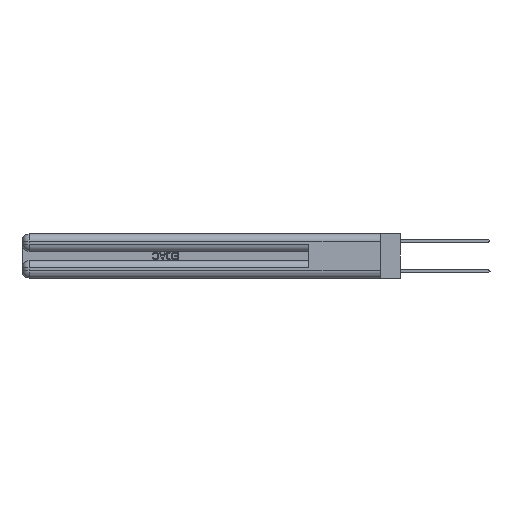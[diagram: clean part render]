
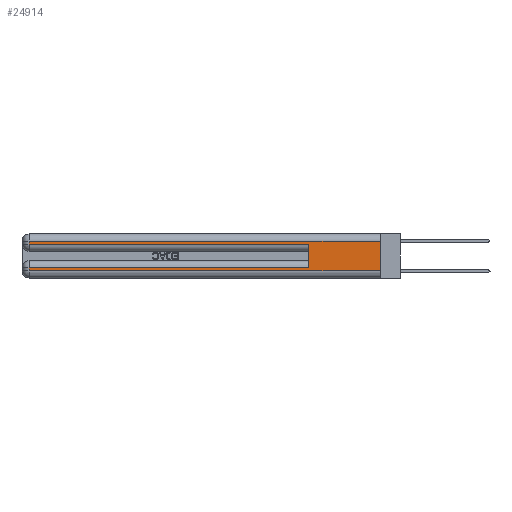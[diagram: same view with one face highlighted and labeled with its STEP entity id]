
A CAD part, left-side view. The second image highlights one B-rep face of the part: STEP entity #24914.
In plain terms, the highlighted planar face has unit normal (-1, 0, 0).
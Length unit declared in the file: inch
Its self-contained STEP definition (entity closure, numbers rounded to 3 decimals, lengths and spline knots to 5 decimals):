
#585 = EDGE_CURVE ( 'NONE', #25290, #20435, #10890, .T. ) ;
#589 = ORIENTED_EDGE ( 'NONE', *, *, #7369, .T. ) ;
#964 = CARTESIAN_POINT ( 'NONE',  ( 0., 0., 0.37 ) ) ;
#1175 = DIRECTION ( 'NONE',  ( 0., 0., -1. ) ) ;
#1409 = LINE ( 'NONE', #19033, #17238 ) ;
#1501 = LINE ( 'NONE', #21539, #28859 ) ;
#2198 = DIRECTION ( 'NONE',  ( 0., 1., 0. ) ) ;
#2528 = CARTESIAN_POINT ( 'NONE',  ( 0., 2.94, 0.06 ) ) ;
#3525 = ORIENTED_EDGE ( 'NONE', *, *, #28565, .T. ) ;
#4118 = CARTESIAN_POINT ( 'NONE',  ( 0., 2.94, 0.37 ) ) ;
#4398 = DIRECTION ( 'NONE',  ( 0., -1., 0. ) ) ;
#4461 = AXIS2_PLACEMENT_3D ( 'NONE', #27944, #15778, #1175 ) ;
#4670 = DIRECTION ( 'NONE',  ( 0., 0., 1. ) ) ;
#5052 = VERTEX_POINT ( 'NONE', #25708 ) ;
#5996 = FACE_OUTER_BOUND ( 'NONE', #27576, .T. ) ;
#6128 = LINE ( 'NONE', #26001, #10800 ) ;
#6422 = CARTESIAN_POINT ( 'NONE',  ( 0., 0., 0.31 ) ) ;
#6440 = DIRECTION ( 'NONE',  ( 0., 0., -1. ) ) ;
#7369 = EDGE_CURVE ( 'NONE', #26856, #5052, #14065, .T. ) ;
#7680 = VECTOR ( 'NONE', #4670, 39.37008 ) ;
#8380 = PLANE ( 'NONE',  #4461 ) ;
#8761 = CARTESIAN_POINT ( 'NONE',  ( 0., 0.6, 0.285 ) ) ;
#9055 = EDGE_CURVE ( 'NONE', #12530, #19710, #1501, .T. ) ;
#9085 = LINE ( 'NONE', #4118, #18811 ) ;
#9588 = EDGE_CURVE ( 'NONE', #26856, #19710, #29171, .T. ) ;
#9983 = EDGE_CURVE ( 'NONE', #5052, #23613, #9085, .T. ) ;
#10800 = VECTOR ( 'NONE', #6440, 39.37008 ) ;
#10890 = LINE ( 'NONE', #964, #15749 ) ;
#12530 = VERTEX_POINT ( 'NONE', #13041 ) ;
#13041 = CARTESIAN_POINT ( 'NONE',  ( 0., 2.94, 0.285 ) ) ;
#13114 = VECTOR ( 'NONE', #2198, 39.37008 ) ;
#13145 = CARTESIAN_POINT ( 'NONE',  ( 0., 0., 0.06 ) ) ;
#14011 = ORIENTED_EDGE ( 'NONE', *, *, #24035, .T. ) ;
#14065 = LINE ( 'NONE', #23860, #13114 ) ;
#14212 = EDGE_CURVE ( 'NONE', #24485, #12530, #6128, .T. ) ;
#14430 = CARTESIAN_POINT ( 'NONE',  ( 0., 0.6, 0.145 ) ) ;
#15690 = CARTESIAN_POINT ( 'NONE',  ( 0., 0., 0.31 ) ) ;
#15749 = VECTOR ( 'NONE', #20044, 39.37008 ) ;
#15778 = DIRECTION ( 'NONE',  ( 1., 0., 0. ) ) ;
#15856 = ORIENTED_EDGE ( 'NONE', *, *, #9588, .F. ) ;
#16626 = ORIENTED_EDGE ( 'NONE', *, *, #14212, .T. ) ;
#17238 = VECTOR ( 'NONE', #21597, 39.37008 ) ;
#17951 = ORIENTED_EDGE ( 'NONE', *, *, #9055, .T. ) ;
#18811 = VECTOR ( 'NONE', #21265, 39.37008 ) ;
#19033 = CARTESIAN_POINT ( 'NONE',  ( 0., 0., 0.06 ) ) ;
#19710 = VERTEX_POINT ( 'NONE', #8761 ) ;
#20044 = DIRECTION ( 'NONE',  ( 0., 0., -1. ) ) ;
#20435 = VERTEX_POINT ( 'NONE', #13145 ) ;
#21265 = DIRECTION ( 'NONE',  ( 0., 0., -1. ) ) ;
#21539 = CARTESIAN_POINT ( 'NONE',  ( 0., 0., 0.285 ) ) ;
#21552 = ORIENTED_EDGE ( 'NONE', *, *, #9983, .T. ) ;
#21597 = DIRECTION ( 'NONE',  ( 0., -1., 0. ) ) ;
#22743 = LINE ( 'NONE', #15690, #30741 ) ;
#23400 = CARTESIAN_POINT ( 'NONE',  ( 0., 0.6, 0.085 ) ) ;
#23613 = VERTEX_POINT ( 'NONE', #2528 ) ;
#23860 = CARTESIAN_POINT ( 'NONE',  ( 0., 0., 0.085 ) ) ;
#24035 = EDGE_CURVE ( 'NONE', #23613, #20435, #1409, .T. ) ;
#24332 = ORIENTED_EDGE ( 'NONE', *, *, #585, .F. ) ;
#24485 = VERTEX_POINT ( 'NONE', #25622 ) ;
#24914 = ADVANCED_FACE ( 'NONE', ( #5996 ), #8380, .F. ) ;
#25290 = VERTEX_POINT ( 'NONE', #6422 ) ;
#25471 = DIRECTION ( 'NONE',  ( 0., 1., 0. ) ) ;
#25622 = CARTESIAN_POINT ( 'NONE',  ( 0., 2.94, 0.31 ) ) ;
#25708 = CARTESIAN_POINT ( 'NONE',  ( 0., 2.94, 0.085 ) ) ;
#26001 = CARTESIAN_POINT ( 'NONE',  ( 0., 2.94, 0.37 ) ) ;
#26856 = VERTEX_POINT ( 'NONE', #23400 ) ;
#27576 = EDGE_LOOP ( 'NONE', ( #24332, #3525, #16626, #17951, #15856, #589, #21552, #14011 ) ) ;
#27944 = CARTESIAN_POINT ( 'NONE',  ( 0., 0., 0.37 ) ) ;
#28565 = EDGE_CURVE ( 'NONE', #25290, #24485, #22743, .T. ) ;
#28859 = VECTOR ( 'NONE', #4398, 39.37008 ) ;
#29171 = LINE ( 'NONE', #14430, #7680 ) ;
#30741 = VECTOR ( 'NONE', #25471, 39.37008 ) ;
